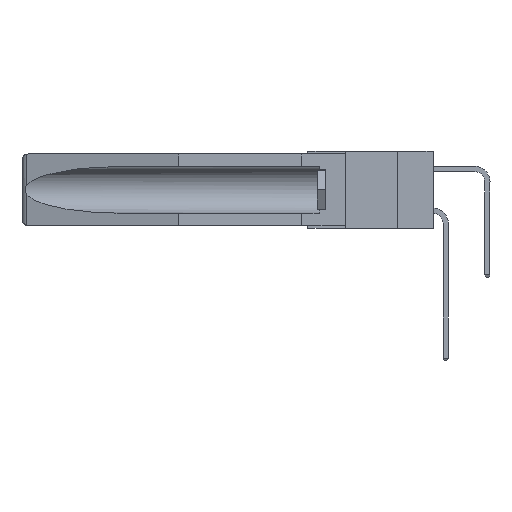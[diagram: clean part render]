
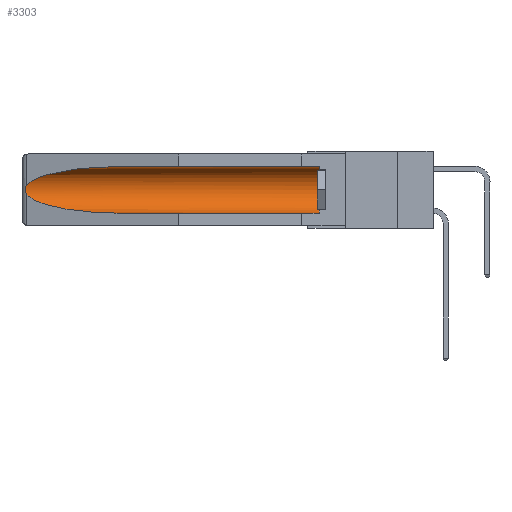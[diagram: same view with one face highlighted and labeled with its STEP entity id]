
A CAD part, left-side view. The second image highlights one B-rep face of the part: STEP entity #3303.
In plain terms, the highlighted cylindrical face has radius 2.857 mm (diameter 5.715 mm), a partial arc.
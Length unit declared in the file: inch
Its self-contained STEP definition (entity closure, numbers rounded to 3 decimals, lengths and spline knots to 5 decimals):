
#52 = DIRECTION ( 'NONE',  ( 0., 1., 0. ) ) ;
#524 = DIRECTION ( 'NONE',  ( 0., 1., 0. ) ) ;
#572 = CARTESIAN_POINT ( 'NONE',  ( 0.26597, 1.5296, -0.19026 ) ) ;
#1486 = ORIENTED_EDGE ( 'NONE', *, *, #14428, .T. ) ;
#1528 = VERTEX_POINT ( 'NONE', #1668 ) ;
#1597 = VECTOR ( 'NONE', #52, 39.37008 ) ;
#1668 = CARTESIAN_POINT ( 'NONE',  ( 0.155, 0.126, -0.284 ) ) ;
#2374 = CARTESIAN_POINT ( 'NONE',  ( 0.26537, 1.52718, -0.19328 ) ) ;
#3303 = ADVANCED_FACE ( 'NONE', ( #24138 ), #16899, .F. ) ;
#3686 = VERTEX_POINT ( 'NONE', #10716 ) ;
#3955 = DIRECTION ( 'NONE',  ( 0., 1., 0. ) ) ;
#4065 = ORIENTED_EDGE ( 'NONE', *, *, #13911, .F. ) ;
#4488 = CARTESIAN_POINT ( 'NONE',  ( 0.155, 0.126, -0.1715 ) ) ;
#4724 = CARTESIAN_POINT ( 'NONE',  ( 0.155, -0.30754, -0.1715 ) ) ;
#4814 =( BOUNDED_CURVE ( )  B_SPLINE_CURVE ( 3, ( #4989, #25065, #7196, #8966 ),
 .UNSPECIFIED., .F., .T. ) 
 B_SPLINE_CURVE_WITH_KNOTS ( ( 4, 4 ),
 ( 0.1948, 1.5708 ),
 .UNSPECIFIED. ) 
 CURVE ( )  GEOMETRIC_REPRESENTATION_ITEM ( )  RATIONAL_B_SPLINE_CURVE ( ( 1., 0.848, 0.848, 1. ) ) 
 REPRESENTATION_ITEM ( '' )  );
#4989 = CARTESIAN_POINT ( 'NONE',  ( 0.26537, 1.52718, -0.19328 ) ) ;
#6317 = EDGE_CURVE ( 'NONE', #8794, #14477, #8410, .T. ) ;
#6585 = AXIS2_PLACEMENT_3D ( 'NONE', #4488, #12157, #18539 ) ;
#6610 = CARTESIAN_POINT ( 'NONE',  ( 0.26655, 1.53094, -0.18657 ) ) ;
#7196 = CARTESIAN_POINT ( 'NONE',  ( 0.21114, 1.30732, -0.284 ) ) ;
#7550 = CARTESIAN_POINT ( 'NONE',  ( 0.26537, 1.52718, -0.14972 ) ) ;
#7970 = CARTESIAN_POINT ( 'NONE',  ( 0.155, -0.30754, -0.284 ) ) ;
#8020 = CARTESIAN_POINT ( 'NONE',  ( 0.26537, 1.52718, -0.14972 ) ) ;
#8323 = CARTESIAN_POINT ( 'NONE',  ( 0.2673, 1.53269, -0.17917 ) ) ;
#8410 = B_SPLINE_CURVE_WITH_KNOTS ( 'NONE', 3,
 ( #10351, #12525, #14266, #16193, #18307, #20330, #8323, #6610, #572, #20670 ),
 .UNSPECIFIED., .F., .F.,
 ( 4, 2, 2, 2, 4 ),
 ( 0., 0.00029, 0.00058, 0.00087, 0.00117 ),
 .UNSPECIFIED. ) ;
#8794 = VERTEX_POINT ( 'NONE', #7550 ) ;
#8966 = CARTESIAN_POINT ( 'NONE',  ( 0.155, 1.07973, -0.284 ) ) ;
#10351 = CARTESIAN_POINT ( 'NONE',  ( 0.26537, 1.52718, -0.14972 ) ) ;
#10716 = CARTESIAN_POINT ( 'NONE',  ( 0.155, 1.07973, -0.059 ) ) ;
#11472 = EDGE_CURVE ( 'NONE', #14477, #23251, #4814, .T. ) ;
#11858 = EDGE_LOOP ( 'NONE', ( #1486, #17928, #13015, #4065, #14980, #18449 ) ) ;
#12157 = DIRECTION ( 'NONE',  ( 0., -1., 0. ) ) ;
#12470 = CARTESIAN_POINT ( 'NONE',  ( 0.155, 1.07973, -0.284 ) ) ;
#12525 = CARTESIAN_POINT ( 'NONE',  ( 0.26597, 1.52961, -0.15275 ) ) ;
#13015 = ORIENTED_EDGE ( 'NONE', *, *, #11472, .T. ) ;
#13911 = EDGE_CURVE ( 'NONE', #1528, #23251, #16675, .T. ) ;
#13977 = CARTESIAN_POINT ( 'NONE',  ( 0.155, 1.07973, -0.059 ) ) ;
#14266 = CARTESIAN_POINT ( 'NONE',  ( 0.26654, 1.53092, -0.15636 ) ) ;
#14428 = EDGE_CURVE ( 'NONE', #3686, #8794, #22390, .T. ) ;
#14477 = VERTEX_POINT ( 'NONE', #2374 ) ;
#14561 = DIRECTION ( 'NONE',  ( 0., 0., 1. ) ) ;
#14980 = ORIENTED_EDGE ( 'NONE', *, *, #21492, .T. ) ;
#15709 = CARTESIAN_POINT ( 'NONE',  ( 0.155, -0.30754, -0.059 ) ) ;
#16193 = CARTESIAN_POINT ( 'NONE',  ( 0.2673, 1.5327, -0.16383 ) ) ;
#16631 = CIRCLE ( 'NONE', #6585, 0.1125 ) ;
#16675 = LINE ( 'NONE', #7970, #1597 ) ;
#16899 = CYLINDRICAL_SURFACE ( 'NONE', #21200, 0.1125 ) ;
#16954 = LINE ( 'NONE', #15709, #23222 ) ;
#17738 = CARTESIAN_POINT ( 'NONE',  ( 0.25451, 1.48313, -0.09465 ) ) ;
#17928 = ORIENTED_EDGE ( 'NONE', *, *, #6317, .T. ) ;
#18307 = CARTESIAN_POINT ( 'NONE',  ( 0.2675, 1.53308, -0.16763 ) ) ;
#18449 = ORIENTED_EDGE ( 'NONE', *, *, #21952, .T. ) ;
#18539 = DIRECTION ( 'NONE',  ( 0., 0., 1. ) ) ;
#20105 = CARTESIAN_POINT ( 'NONE',  ( 0.21114, 1.30732, -0.059 ) ) ;
#20330 = CARTESIAN_POINT ( 'NONE',  ( 0.2675, 1.53308, -0.17534 ) ) ;
#20670 = CARTESIAN_POINT ( 'NONE',  ( 0.26537, 1.52718, -0.19328 ) ) ;
#21200 = AXIS2_PLACEMENT_3D ( 'NONE', #4724, #524, #14561 ) ;
#21492 = EDGE_CURVE ( 'NONE', #1528, #23800, #16631, .T. ) ;
#21952 = EDGE_CURVE ( 'NONE', #23800, #3686, #16954, .T. ) ;
#22390 =( BOUNDED_CURVE ( )  B_SPLINE_CURVE ( 3, ( #13977, #20105, #17738, #8020 ),
 .UNSPECIFIED., .F., .F. ) 
 B_SPLINE_CURVE_WITH_KNOTS ( ( 4, 4 ),
 ( 4.71239, 6.08839 ),
 .UNSPECIFIED. ) 
 CURVE ( )  GEOMETRIC_REPRESENTATION_ITEM ( )  RATIONAL_B_SPLINE_CURVE ( ( 1., 0.848, 0.848, 1. ) ) 
 REPRESENTATION_ITEM ( '' )  );
#23222 = VECTOR ( 'NONE', #3955, 39.37008 ) ;
#23251 = VERTEX_POINT ( 'NONE', #12470 ) ;
#23800 = VERTEX_POINT ( 'NONE', #23860 ) ;
#23860 = CARTESIAN_POINT ( 'NONE',  ( 0.155, 0.126, -0.059 ) ) ;
#24138 = FACE_OUTER_BOUND ( 'NONE', #11858, .T. ) ;
#25065 = CARTESIAN_POINT ( 'NONE',  ( 0.25451, 1.48313, -0.24835 ) ) ;
